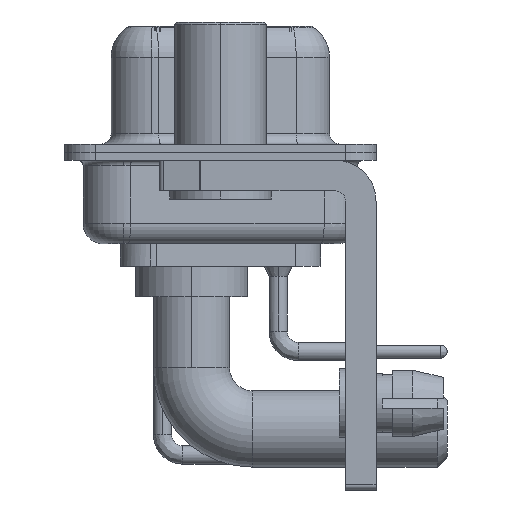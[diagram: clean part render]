
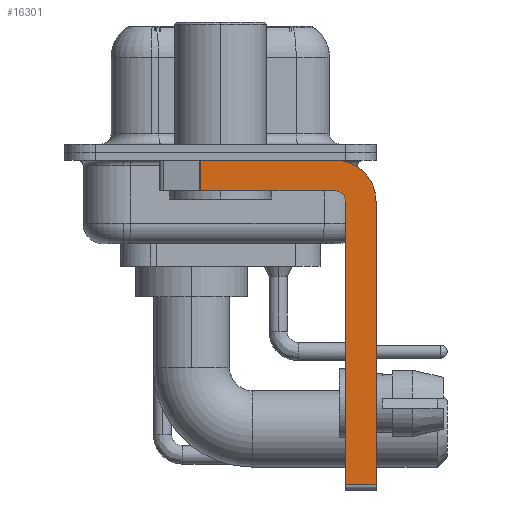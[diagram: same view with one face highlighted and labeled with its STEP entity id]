
A CAD part, left-side view. The second image highlights one B-rep face of the part: STEP entity #16301.
In plain terms, the highlighted planar face has unit normal (-1, 0, 0).
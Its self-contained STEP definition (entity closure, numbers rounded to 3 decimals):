
#83 = DIRECTION ( 'NONE',  ( 0., -1., 0. ) ) ;
#279 = DIRECTION ( 'NONE',  ( 1., 0., 0. ) ) ;
#310 = AXIS2_PLACEMENT_3D ( 'NONE', #23197, #32030, #22805 ) ;
#1201 = LINE ( 'NONE', #22194, #37543 ) ;
#1834 = DIRECTION ( 'NONE',  ( 0., 0., 1. ) ) ;
#2063 = ORIENTED_EDGE ( 'NONE', *, *, #16049, .F. ) ;
#2183 = FACE_OUTER_BOUND ( 'NONE', #33463, .T. ) ;
#2311 = ORIENTED_EDGE ( 'NONE', *, *, #19112, .F. ) ;
#4051 = DIRECTION ( 'NONE',  ( 0., 0., -1. ) ) ;
#4164 = CARTESIAN_POINT ( 'NONE',  ( -2.9, -5.65, -0.4 ) ) ;
#4582 = VECTOR ( 'NONE', #32079, 1000. ) ;
#5820 = LINE ( 'NONE', #17563, #10680 ) ;
#5847 = DIRECTION ( 'NONE',  ( -1., 0., 0. ) ) ;
#5852 = LINE ( 'NONE', #13934, #33974 ) ;
#9336 = ORIENTED_EDGE ( 'NONE', *, *, #26861, .F. ) ;
#10680 = VECTOR ( 'NONE', #4051, 1000. ) ;
#12209 = DIRECTION ( 'NONE',  ( 0., 0., 1. ) ) ;
#12549 = ORIENTED_EDGE ( 'NONE', *, *, #27902, .T. ) ;
#12633 = DIRECTION ( 'NONE',  ( 0., 0., -1. ) ) ;
#12765 = CIRCLE ( 'NONE', #31833, 0.5 ) ;
#13934 = CARTESIAN_POINT ( 'NONE',  ( -2.9, 3., -0.4 ) ) ;
#14082 = VERTEX_POINT ( 'NONE', #16156 ) ;
#14238 = VERTEX_POINT ( 'NONE', #23283 ) ;
#15796 = ORIENTED_EDGE ( 'NONE', *, *, #34431, .F. ) ;
#16049 = EDGE_CURVE ( 'NONE', #27763, #25710, #31896, .T. ) ;
#16156 = CARTESIAN_POINT ( 'NONE',  ( -2.9, -7.65, -2.4 ) ) ;
#16301 = ADVANCED_FACE ( 'NONE', ( #2183 ), #29142, .F. ) ;
#17090 = ORIENTED_EDGE ( 'NONE', *, *, #19694, .F. ) ;
#17320 = ORIENTED_EDGE ( 'NONE', *, *, #36384, .F. ) ;
#17442 = LINE ( 'NONE', #25518, #28715 ) ;
#17560 = VERTEX_POINT ( 'NONE', #4164 ) ;
#17563 = CARTESIAN_POINT ( 'NONE',  ( -2.9, -7.65, -2.4 ) ) ;
#18504 = CARTESIAN_POINT ( 'NONE',  ( -2.9, 0.978, -0.4 ) ) ;
#18764 = CARTESIAN_POINT ( 'NONE',  ( -2.9, 0.978, -1.9 ) ) ;
#19021 = CIRCLE ( 'NONE', #28244, 2. ) ;
#19112 = EDGE_CURVE ( 'NONE', #19120, #14238, #17442, .T. ) ;
#19120 = VERTEX_POINT ( 'NONE', #25327 ) ;
#19694 = EDGE_CURVE ( 'NONE', #14238, #27763, #12765, .T. ) ;
#21220 = CARTESIAN_POINT ( 'NONE',  ( -2.9, -7.65, -16.35 ) ) ;
#21296 = CARTESIAN_POINT ( 'NONE',  ( -2.9, -5.65, -2.4 ) ) ;
#22194 = CARTESIAN_POINT ( 'NONE',  ( -2.9, 0.978, -1.9 ) ) ;
#22805 = DIRECTION ( 'NONE',  ( 0., 0., -1. ) ) ;
#23197 = CARTESIAN_POINT ( 'NONE',  ( -2.9, -5.65, -2.4 ) ) ;
#23283 = CARTESIAN_POINT ( 'NONE',  ( -2.9, -6.15, -2.4 ) ) ;
#23379 = DIRECTION ( 'NONE',  ( 0., -1., 0. ) ) ;
#23748 = CARTESIAN_POINT ( 'NONE',  ( -2.9, -5.65, -2.4 ) ) ;
#24525 = DIRECTION ( 'NONE',  ( 0., 0., -1. ) ) ;
#24808 = CARTESIAN_POINT ( 'NONE',  ( -2.9, -5.65, -1.9 ) ) ;
#25327 = CARTESIAN_POINT ( 'NONE',  ( -2.9, -6.15, -16.35 ) ) ;
#25518 = CARTESIAN_POINT ( 'NONE',  ( -2.9, -6.15, -16.6 ) ) ;
#25710 = VERTEX_POINT ( 'NONE', #18764 ) ;
#26112 = CARTESIAN_POINT ( 'NONE',  ( -2.9, -5.65, -1.9 ) ) ;
#26861 = EDGE_CURVE ( 'NONE', #17560, #14082, #19021, .T. ) ;
#27763 = VERTEX_POINT ( 'NONE', #24808 ) ;
#27865 = ORIENTED_EDGE ( 'NONE', *, *, #33985, .T. ) ;
#27902 = EDGE_CURVE ( 'NONE', #37572, #25710, #1201, .T. ) ;
#28244 = AXIS2_PLACEMENT_3D ( 'NONE', #21296, #279, #12633 ) ;
#28715 = VECTOR ( 'NONE', #1834, 1000. ) ;
#28995 = CARTESIAN_POINT ( 'NONE',  ( -2.9, -5.65, -16.35 ) ) ;
#29142 = PLANE ( 'NONE',  #310 ) ;
#29513 = VERTEX_POINT ( 'NONE', #21220 ) ;
#31833 = AXIS2_PLACEMENT_3D ( 'NONE', #23748, #5847, #12209 ) ;
#31896 = LINE ( 'NONE', #26112, #4582 ) ;
#32030 = DIRECTION ( 'NONE',  ( 1., 0., 0. ) ) ;
#32079 = DIRECTION ( 'NONE',  ( 0., 1., 0. ) ) ;
#33463 = EDGE_LOOP ( 'NONE', ( #15796, #12549, #2063, #17090, #2311, #27865, #17320, #9336 ) ) ;
#33974 = VECTOR ( 'NONE', #23379, 1000. ) ;
#33985 = EDGE_CURVE ( 'NONE', #19120, #29513, #37870, .T. ) ;
#34431 = EDGE_CURVE ( 'NONE', #37572, #17560, #5852, .T. ) ;
#36384 = EDGE_CURVE ( 'NONE', #14082, #29513, #5820, .T. ) ;
#37543 = VECTOR ( 'NONE', #24525, 1000. ) ;
#37572 = VERTEX_POINT ( 'NONE', #18504 ) ;
#37677 = VECTOR ( 'NONE', #83, 1000. ) ;
#37870 = LINE ( 'NONE', #28995, #37677 ) ;
